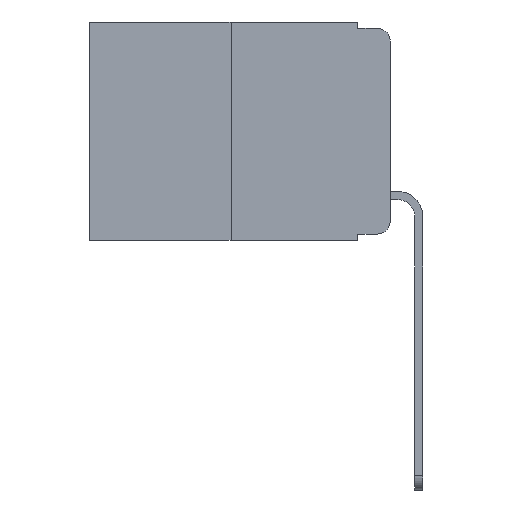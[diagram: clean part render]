
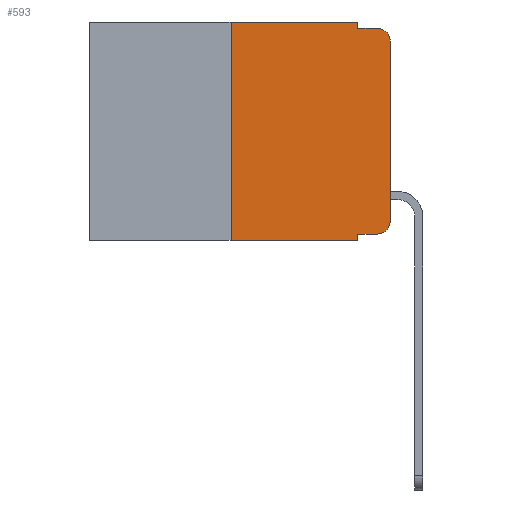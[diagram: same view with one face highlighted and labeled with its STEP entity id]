
A CAD part, left-side view. The second image highlights one B-rep face of the part: STEP entity #593.
In plain terms, the highlighted planar face has unit normal (-1, 0, 0).
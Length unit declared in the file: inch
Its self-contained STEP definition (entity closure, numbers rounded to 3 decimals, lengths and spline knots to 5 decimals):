
#15 = LINE ( 'NONE', #3165, #18037 ) ;
#53 = ORIENTED_EDGE ( 'NONE', *, *, #13283, .F. ) ;
#244 = LINE ( 'NONE', #4499, #15927 ) ;
#443 = LINE ( 'NONE', #1732, #19187 ) ;
#453 = VERTEX_POINT ( 'NONE', #5974 ) ;
#525 = VERTEX_POINT ( 'NONE', #10453 ) ;
#593 = ADVANCED_FACE ( 'NONE', ( #2954 ), #10337, .F. ) ;
#595 = VERTEX_POINT ( 'NONE', #12928 ) ;
#616 = VERTEX_POINT ( 'NONE', #6557 ) ;
#672 = ORIENTED_EDGE ( 'NONE', *, *, #3863, .F. ) ;
#1051 = VERTEX_POINT ( 'NONE', #14820 ) ;
#1062 = VERTEX_POINT ( 'NONE', #8172 ) ;
#1147 = CARTESIAN_POINT ( 'NONE',  ( 0., 0.051, 0. ) ) ;
#1381 = DIRECTION ( 'NONE',  ( 0., 0., -1. ) ) ;
#1640 = ORIENTED_EDGE ( 'NONE', *, *, #18342, .F. ) ;
#1732 = CARTESIAN_POINT ( 'NONE',  ( 0., 0.473, -0.343 ) ) ;
#2149 = DIRECTION ( 'NONE',  ( 0., 0., 1. ) ) ;
#2312 = ORIENTED_EDGE ( 'NONE', *, *, #11417, .T. ) ;
#2403 = ORIENTED_EDGE ( 'NONE', *, *, #7840, .F. ) ;
#2646 = LINE ( 'NONE', #19007, #10461 ) ;
#2702 = DIRECTION ( 'NONE',  ( 0., -1., 0. ) ) ;
#2939 = ORIENTED_EDGE ( 'NONE', *, *, #13430, .T. ) ;
#2954 = FACE_OUTER_BOUND ( 'NONE', #12943, .T. ) ;
#2977 = ORIENTED_EDGE ( 'NONE', *, *, #6930, .F. ) ;
#3165 = CARTESIAN_POINT ( 'NONE',  ( 0., 0.051, 0. ) ) ;
#3414 = ORIENTED_EDGE ( 'NONE', *, *, #7318, .T. ) ;
#3458 = ORIENTED_EDGE ( 'NONE', *, *, #7255, .T. ) ;
#3863 = EDGE_CURVE ( 'NONE', #13699, #616, #15, .T. ) ;
#4499 = CARTESIAN_POINT ( 'NONE',  ( 0., 0.473, 0. ) ) ;
#4752 = VERTEX_POINT ( 'NONE', #8311 ) ;
#5599 = ORIENTED_EDGE ( 'NONE', *, *, #12354, .T. ) ;
#5677 = VECTOR ( 'NONE', #9228, 39.37008 ) ;
#5878 = CARTESIAN_POINT ( 'NONE',  ( 0., 0.25, 0. ) ) ;
#5893 = LINE ( 'NONE', #5878, #9895 ) ;
#5974 = CARTESIAN_POINT ( 'NONE',  ( 0., 0.25, 0. ) ) ;
#6436 = AXIS2_PLACEMENT_3D ( 'NONE', #7457, #17194, #8896 ) ;
#6557 = CARTESIAN_POINT ( 'NONE',  ( 0., 0.051, -0.01 ) ) ;
#6930 = EDGE_CURVE ( 'NONE', #8299, #4752, #9713, .T. ) ;
#6955 = AXIS2_PLACEMENT_3D ( 'NONE', #11736, #14709, #7597 ) ;
#7255 = EDGE_CURVE ( 'NONE', #595, #17272, #13420, .T. ) ;
#7318 = EDGE_CURVE ( 'NONE', #8299, #595, #8326, .T. ) ;
#7457 = CARTESIAN_POINT ( 'NONE',  ( 0., 0.02, -0.313 ) ) ;
#7597 = DIRECTION ( 'NONE',  ( 0., 0., -1. ) ) ;
#7790 = VECTOR ( 'NONE', #2149, 39.37008 ) ;
#7840 = EDGE_CURVE ( 'NONE', #525, #453, #5893, .T. ) ;
#8172 = CARTESIAN_POINT ( 'NONE',  ( 0., 0.02, -0.01 ) ) ;
#8299 = VERTEX_POINT ( 'NONE', #17274 ) ;
#8311 = CARTESIAN_POINT ( 'NONE',  ( 0., 0.051, -0.343 ) ) ;
#8326 = LINE ( 'NONE', #11887, #18911 ) ;
#8896 = DIRECTION ( 'NONE',  ( 0., 0., -1. ) ) ;
#9228 = DIRECTION ( 'NONE',  ( 0., 0., -1. ) ) ;
#9713 = LINE ( 'NONE', #1147, #5677 ) ;
#9775 = CIRCLE ( 'NONE', #12553, 0.02 ) ;
#9895 = VECTOR ( 'NONE', #18522, 39.37008 ) ;
#10005 = CARTESIAN_POINT ( 'NONE',  ( 0., 0., 0. ) ) ;
#10337 = PLANE ( 'NONE',  #6955 ) ;
#10453 = CARTESIAN_POINT ( 'NONE',  ( 0., 0.25, -0.343 ) ) ;
#10461 = VECTOR ( 'NONE', #17722, 39.37008 ) ;
#10805 = DIRECTION ( 'NONE',  ( -1., 0., 0. ) ) ;
#11417 = EDGE_CURVE ( 'NONE', #17272, #1051, #12204, .T. ) ;
#11736 = CARTESIAN_POINT ( 'NONE',  ( 0., 0.473, 0. ) ) ;
#11887 = CARTESIAN_POINT ( 'NONE',  ( 0., 0.051, -0.333 ) ) ;
#12020 = DIRECTION ( 'NONE',  ( 0., -1., 0. ) ) ;
#12204 = LINE ( 'NONE', #10005, #7790 ) ;
#12354 = EDGE_CURVE ( 'NONE', #1051, #1062, #9775, .T. ) ;
#12553 = AXIS2_PLACEMENT_3D ( 'NONE', #18957, #10805, #1381 ) ;
#12829 = CARTESIAN_POINT ( 'NONE',  ( 0., 0.051, 0. ) ) ;
#12928 = CARTESIAN_POINT ( 'NONE',  ( 0., 0.02, -0.333 ) ) ;
#12943 = EDGE_LOOP ( 'NONE', ( #2312, #5599, #53, #672, #1640, #2403, #2939, #2977, #3414, #3458 ) ) ;
#13283 = EDGE_CURVE ( 'NONE', #616, #1062, #2646, .T. ) ;
#13420 = CIRCLE ( 'NONE', #6436, 0.02 ) ;
#13430 = EDGE_CURVE ( 'NONE', #525, #4752, #443, .T. ) ;
#13537 = CARTESIAN_POINT ( 'NONE',  ( 0., 0., -0.313 ) ) ;
#13699 = VERTEX_POINT ( 'NONE', #12829 ) ;
#14709 = DIRECTION ( 'NONE',  ( 1., 0., 0. ) ) ;
#14820 = CARTESIAN_POINT ( 'NONE',  ( 0., 0., -0.03 ) ) ;
#15927 = VECTOR ( 'NONE', #12020, 39.37008 ) ;
#16405 = DIRECTION ( 'NONE',  ( 0., 0., -1. ) ) ;
#16547 = DIRECTION ( 'NONE',  ( 0., -1., 0. ) ) ;
#17194 = DIRECTION ( 'NONE',  ( -1., 0., 0. ) ) ;
#17272 = VERTEX_POINT ( 'NONE', #13537 ) ;
#17274 = CARTESIAN_POINT ( 'NONE',  ( 0., 0.051, -0.333 ) ) ;
#17722 = DIRECTION ( 'NONE',  ( 0., -1., 0. ) ) ;
#18037 = VECTOR ( 'NONE', #16405, 39.37008 ) ;
#18342 = EDGE_CURVE ( 'NONE', #453, #13699, #244, .T. ) ;
#18522 = DIRECTION ( 'NONE',  ( 0., 0., 1. ) ) ;
#18911 = VECTOR ( 'NONE', #2702, 39.37008 ) ;
#18957 = CARTESIAN_POINT ( 'NONE',  ( 0., 0.02, -0.03 ) ) ;
#19007 = CARTESIAN_POINT ( 'NONE',  ( 0., 0.051, -0.01 ) ) ;
#19187 = VECTOR ( 'NONE', #16547, 39.37008 ) ;
